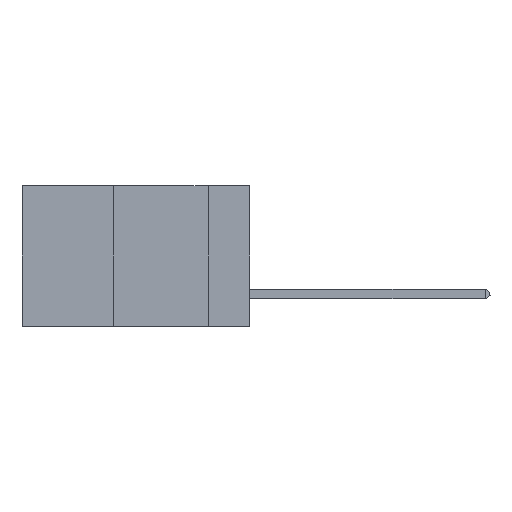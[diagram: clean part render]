
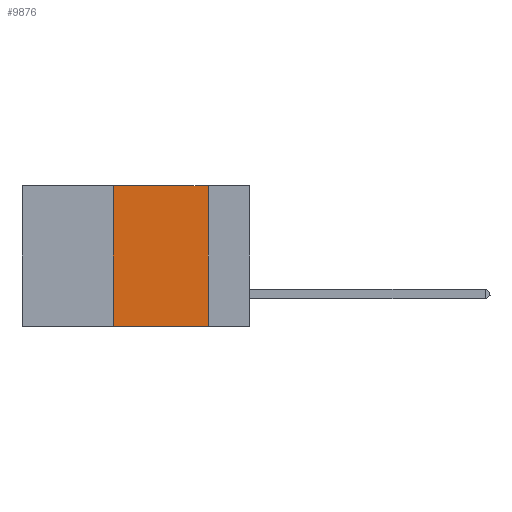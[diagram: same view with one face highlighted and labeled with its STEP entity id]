
A CAD part, left-side view. The second image highlights one B-rep face of the part: STEP entity #9876.
In plain terms, the highlighted planar face has unit normal (-1, 0, 0).
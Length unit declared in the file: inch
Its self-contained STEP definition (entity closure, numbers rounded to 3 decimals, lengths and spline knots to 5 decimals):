
#399 = CARTESIAN_POINT ( 'NONE',  ( 0., 0.6, -0.37 ) ) ;
#405 = VERTEX_POINT ( 'NONE', #10165 ) ;
#1426 = CARTESIAN_POINT ( 'NONE',  ( 0., 0.6, 0. ) ) ;
#1466 = EDGE_LOOP ( 'NONE', ( #8645, #2178, #10919, #4816 ) ) ;
#1599 = CARTESIAN_POINT ( 'NONE',  ( 0., 0.11, 0. ) ) ;
#2178 = ORIENTED_EDGE ( 'NONE', *, *, #3396, .F. ) ;
#2379 = EDGE_CURVE ( 'NONE', #5417, #405, #7749, .T. ) ;
#3396 = EDGE_CURVE ( 'NONE', #10868, #5417, #4016, .T. ) ;
#3587 = CARTESIAN_POINT ( 'NONE',  ( 0., 0.36, -0.37 ) ) ;
#4016 = LINE ( 'NONE', #1426, #6187 ) ;
#4032 = DIRECTION ( 'NONE',  ( 0., 0., 1. ) ) ;
#4503 = DIRECTION ( 'NONE',  ( 1., 0., 0. ) ) ;
#4816 = ORIENTED_EDGE ( 'NONE', *, *, #8106, .T. ) ;
#5307 = PLANE ( 'NONE',  #9260 ) ;
#5417 = VERTEX_POINT ( 'NONE', #9763 ) ;
#5744 = VERTEX_POINT ( 'NONE', #3587 ) ;
#5794 = DIRECTION ( 'NONE',  ( 0., -1., 0. ) ) ;
#5907 = VECTOR ( 'NONE', #4032, 39.37008 ) ;
#6187 = VECTOR ( 'NONE', #8326, 39.37008 ) ;
#6758 = CARTESIAN_POINT ( 'NONE',  ( 0., 0.36, 0. ) ) ;
#6894 = FACE_OUTER_BOUND ( 'NONE', #1466, .T. ) ;
#6999 = DIRECTION ( 'NONE',  ( 0., 0., -1. ) ) ;
#7542 = LINE ( 'NONE', #9290, #5907 ) ;
#7749 = LINE ( 'NONE', #1599, #10484 ) ;
#8106 = EDGE_CURVE ( 'NONE', #5744, #405, #10483, .T. ) ;
#8165 = VECTOR ( 'NONE', #5794, 39.37008 ) ;
#8326 = DIRECTION ( 'NONE',  ( 0., -1., 0. ) ) ;
#8645 = ORIENTED_EDGE ( 'NONE', *, *, #2379, .F. ) ;
#8833 = CARTESIAN_POINT ( 'NONE',  ( 0., 0.6, 0. ) ) ;
#9260 = AXIS2_PLACEMENT_3D ( 'NONE', #8833, #4503, #6999 ) ;
#9290 = CARTESIAN_POINT ( 'NONE',  ( 0., 0.36, 0. ) ) ;
#9586 = DIRECTION ( 'NONE',  ( 0., 0., -1. ) ) ;
#9763 = CARTESIAN_POINT ( 'NONE',  ( 0., 0.11, 0. ) ) ;
#9876 = ADVANCED_FACE ( 'NONE', ( #6894 ), #5307, .F. ) ;
#10165 = CARTESIAN_POINT ( 'NONE',  ( 0., 0.11, -0.37 ) ) ;
#10483 = LINE ( 'NONE', #399, #8165 ) ;
#10484 = VECTOR ( 'NONE', #9586, 39.37008 ) ;
#10868 = VERTEX_POINT ( 'NONE', #6758 ) ;
#10919 = ORIENTED_EDGE ( 'NONE', *, *, #11263, .F. ) ;
#11263 = EDGE_CURVE ( 'NONE', #5744, #10868, #7542, .T. ) ;
